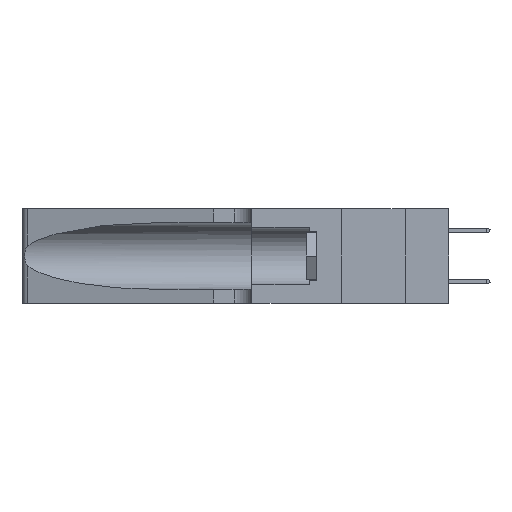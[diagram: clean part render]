
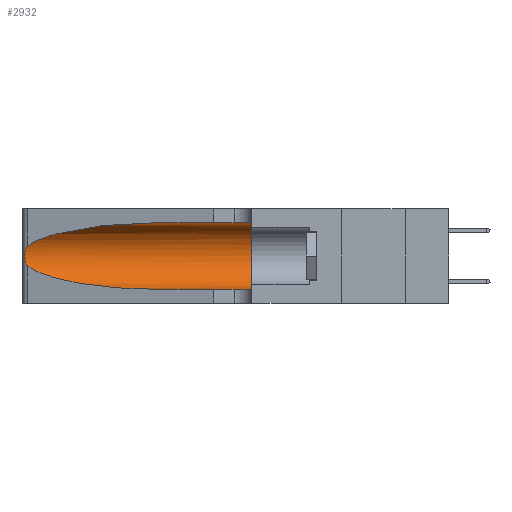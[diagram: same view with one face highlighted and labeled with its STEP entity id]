
A CAD part, left-side view. The second image highlights one B-rep face of the part: STEP entity #2932.
In plain terms, the highlighted cylindrical face has radius 3.308 mm (diameter 6.617 mm), a partial arc.
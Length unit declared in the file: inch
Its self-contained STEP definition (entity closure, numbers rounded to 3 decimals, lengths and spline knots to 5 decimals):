
#44 =( BOUNDED_CURVE ( )  B_SPLINE_CURVE ( 3, ( #20491, #12808, #14740, #5010 ),
 .UNSPECIFIED., .F., .T. ) 
 B_SPLINE_CURVE_WITH_KNOTS ( ( 4, 4 ),
 ( 1.5708, 2.84003 ),
 .UNSPECIFIED. ) 
 CURVE ( )  GEOMETRIC_REPRESENTATION_ITEM ( )  RATIONAL_B_SPLINE_CURVE ( ( 1., 0.87, 0.87, 1. ) ) 
 REPRESENTATION_ITEM ( '' )  );
#137 = CARTESIAN_POINT ( 'NONE',  ( 0.25487, 1.22718, 0.14631 ) ) ;
#220 = CARTESIAN_POINT ( 'NONE',  ( 0.25639, 1.23186, 0.15144 ) ) ;
#1763 = DIRECTION ( 'NONE',  ( 0., 0., 1. ) ) ;
#1773 = DIRECTION ( 'NONE',  ( 0., 0., -1. ) ) ;
#1870 = CARTESIAN_POINT ( 'NONE',  ( 0.25487, 1.22718, 0.14631 ) ) ;
#2932 = ADVANCED_FACE ( 'NONE', ( #4901 ), #6081, .F. ) ;
#2981 = VERTEX_POINT ( 'NONE', #24900 ) ;
#3354 = CARTESIAN_POINT ( 'NONE',  ( 0.25555, 1.22994, 0.2215 ) ) ;
#3436 = CARTESIAN_POINT ( 'NONE',  ( 0.25787, 1.23484, 0.2124 ) ) ;
#3758 = VERTEX_POINT ( 'NONE', #17596 ) ;
#4011 = CARTESIAN_POINT ( 'NONE',  ( 0.25555, 1.22993, 0.14849 ) ) ;
#4017 = ORIENTED_EDGE ( 'NONE', *, *, #17477, .F. ) ;
#4446 = CARTESIAN_POINT ( 'NONE',  ( 0.18966, 0.96281, 0.05475 ) ) ;
#4901 = FACE_OUTER_BOUND ( 'NONE', #15162, .T. ) ;
#4948 = VECTOR ( 'NONE', #24355, 39.37008 ) ;
#5010 = CARTESIAN_POINT ( 'NONE',  ( 0.25487, 1.22718, 0.22369 ) ) ;
#5263 = DIRECTION ( 'NONE',  ( 0., 1., 0. ) ) ;
#5746 = CARTESIAN_POINT ( 'NONE',  ( 0.26017, 1.23833, 0.17102 ) ) ;
#6081 = CYLINDRICAL_SURFACE ( 'NONE', #10963, 0.13025 ) ;
#6811 = LINE ( 'NONE', #16029, #14052 ) ;
#7169 = CARTESIAN_POINT ( 'NONE',  ( 0.25639, 1.23184, 0.21858 ) ) ;
#7559 = CARTESIAN_POINT ( 'NONE',  ( 0.1305, 0.35, 0.31525 ) ) ;
#7680 = CARTESIAN_POINT ( 'NONE',  ( 0.25856, 1.23593, 0.16098 ) ) ;
#7685 = B_SPLINE_CURVE_WITH_KNOTS ( 'NONE', 3,
 ( #12908, #3354, #7169, #3436, #9128, #20767, #11137, #15017, #5746, #7680, #11637, #220, #4011, #137 ),
 .UNSPECIFIED., .F., .F.,
 ( 4, 2, 2, 2, 2, 2, 4 ),
 ( 0., 0.00027, 0.00053, 0.00107, 0.0016, 0.00187, 0.00214 ),
 .UNSPECIFIED. ) ;
#7743 = CARTESIAN_POINT ( 'NONE',  ( 0.1305, 0.35, 0.05475 ) ) ;
#8380 = CARTESIAN_POINT ( 'NONE',  ( 0.2373, 1.15595, 0.08982 ) ) ;
#9128 = CARTESIAN_POINT ( 'NONE',  ( 0.25854, 1.2359, 0.20912 ) ) ;
#10029 = LINE ( 'NONE', #18802, #4948 ) ;
#10963 = AXIS2_PLACEMENT_3D ( 'NONE', #13405, #13244, #1773 ) ;
#11137 = CARTESIAN_POINT ( 'NONE',  ( 0.26075, 1.23896, 0.19203 ) ) ;
#11535 = ORIENTED_EDGE ( 'NONE', *, *, #23541, .T. ) ;
#11637 = CARTESIAN_POINT ( 'NONE',  ( 0.25789, 1.23486, 0.15765 ) ) ;
#12123 = DIRECTION ( 'NONE',  ( 0., -1., 0. ) ) ;
#12808 = CARTESIAN_POINT ( 'NONE',  ( 0.18966, 0.96281, 0.31525 ) ) ;
#12908 = CARTESIAN_POINT ( 'NONE',  ( 0.25487, 1.22718, 0.22369 ) ) ;
#13102 = VERTEX_POINT ( 'NONE', #7559 ) ;
#13244 = DIRECTION ( 'NONE',  ( 0., -1., 0. ) ) ;
#13405 = CARTESIAN_POINT ( 'NONE',  ( 0.1305, 1.61858, 0.185 ) ) ;
#14052 = VECTOR ( 'NONE', #12123, 39.37008 ) ;
#14740 = CARTESIAN_POINT ( 'NONE',  ( 0.2373, 1.15595, 0.28018 ) ) ;
#15017 = CARTESIAN_POINT ( 'NONE',  ( 0.26075, 1.23896, 0.178 ) ) ;
#15162 = EDGE_LOOP ( 'NONE', ( #21721, #11535, #18970, #19399, #4017, #18792 ) ) ;
#15755 = VERTEX_POINT ( 'NONE', #1870 ) ;
#16029 = CARTESIAN_POINT ( 'NONE',  ( 0.1305, 1.61858, 0.05475 ) ) ;
#16135 = CARTESIAN_POINT ( 'NONE',  ( 0.1305, 0.72297, 0.05475 ) ) ;
#16290 = EDGE_CURVE ( 'NONE', #22150, #3758, #44, .T. ) ;
#16583 = VERTEX_POINT ( 'NONE', #7743 ) ;
#17477 = EDGE_CURVE ( 'NONE', #13102, #16583, #21237, .T. ) ;
#17596 = CARTESIAN_POINT ( 'NONE',  ( 0.25487, 1.22718, 0.22369 ) ) ;
#18144 = EDGE_CURVE ( 'NONE', #22150, #13102, #10029, .T. ) ;
#18234 = CARTESIAN_POINT ( 'NONE',  ( 0.25487, 1.22718, 0.14631 ) ) ;
#18792 = ORIENTED_EDGE ( 'NONE', *, *, #18144, .F. ) ;
#18802 = CARTESIAN_POINT ( 'NONE',  ( 0.1305, 1.61858, 0.31525 ) ) ;
#18970 = ORIENTED_EDGE ( 'NONE', *, *, #23233, .T. ) ;
#19399 = ORIENTED_EDGE ( 'NONE', *, *, #23754, .T. ) ;
#20491 = CARTESIAN_POINT ( 'NONE',  ( 0.1305, 0.72297, 0.31525 ) ) ;
#20767 = CARTESIAN_POINT ( 'NONE',  ( 0.26018, 1.23835, 0.19895 ) ) ;
#21237 = CIRCLE ( 'NONE', #21487, 0.13025 ) ;
#21487 = AXIS2_PLACEMENT_3D ( 'NONE', #24640, #5263, #1763 ) ;
#21721 = ORIENTED_EDGE ( 'NONE', *, *, #16290, .T. ) ;
#22150 = VERTEX_POINT ( 'NONE', #23742 ) ;
#22673 =( BOUNDED_CURVE ( )  B_SPLINE_CURVE ( 3, ( #18234, #8380, #4446, #16135 ),
 .UNSPECIFIED., .F., .T. ) 
 B_SPLINE_CURVE_WITH_KNOTS ( ( 4, 4 ),
 ( 3.44316, 4.71239 ),
 .UNSPECIFIED. ) 
 CURVE ( )  GEOMETRIC_REPRESENTATION_ITEM ( )  RATIONAL_B_SPLINE_CURVE ( ( 1., 0.87, 0.87, 1. ) ) 
 REPRESENTATION_ITEM ( '' )  );
#23233 = EDGE_CURVE ( 'NONE', #15755, #2981, #22673, .T. ) ;
#23541 = EDGE_CURVE ( 'NONE', #3758, #15755, #7685, .T. ) ;
#23742 = CARTESIAN_POINT ( 'NONE',  ( 0.1305, 0.72297, 0.31525 ) ) ;
#23754 = EDGE_CURVE ( 'NONE', #2981, #16583, #6811, .T. ) ;
#24355 = DIRECTION ( 'NONE',  ( 0., -1., 0. ) ) ;
#24640 = CARTESIAN_POINT ( 'NONE',  ( 0.1305, 0.35, 0.185 ) ) ;
#24900 = CARTESIAN_POINT ( 'NONE',  ( 0.1305, 0.72297, 0.05475 ) ) ;
